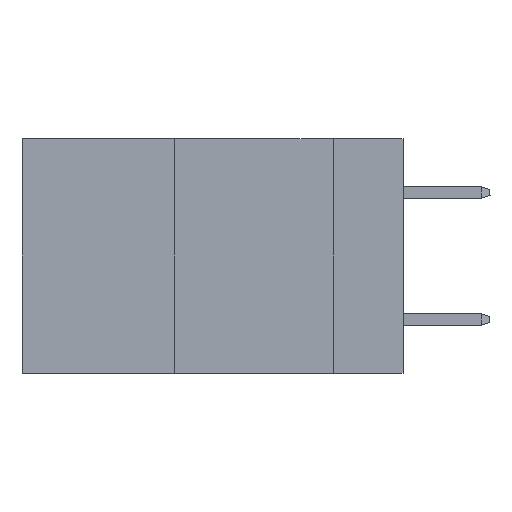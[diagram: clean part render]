
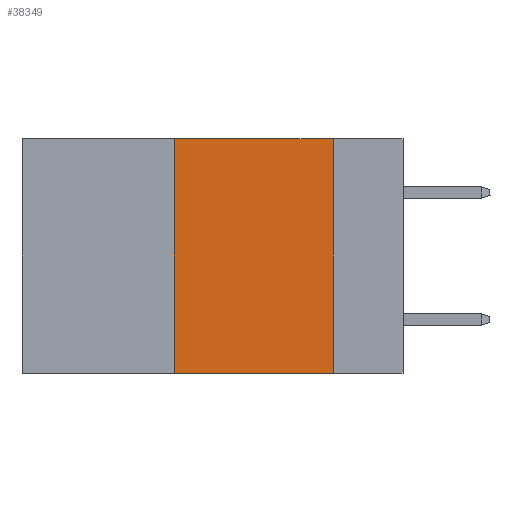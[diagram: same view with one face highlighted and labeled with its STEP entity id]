
A CAD part, left-side view. The second image highlights one B-rep face of the part: STEP entity #38349.
In plain terms, the highlighted planar face has unit normal (-1, 0, 0).
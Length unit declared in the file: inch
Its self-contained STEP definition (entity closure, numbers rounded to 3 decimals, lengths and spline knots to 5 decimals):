
#285 = ORIENTED_EDGE ( 'NONE', *, *, #9328, .T. ) ;
#897 = CARTESIAN_POINT ( 'NONE',  ( 0., 0.11, 0. ) ) ;
#1718 = VECTOR ( 'NONE', #2829, 39.37008 ) ;
#2829 = DIRECTION ( 'NONE',  ( 0., -1., 0. ) ) ;
#4061 = DIRECTION ( 'NONE',  ( 1., 0., 0. ) ) ;
#5823 = DIRECTION ( 'NONE',  ( 0., 0., 1. ) ) ;
#6064 = CARTESIAN_POINT ( 'NONE',  ( 0., 0.36, 0. ) ) ;
#6321 = VERTEX_POINT ( 'NONE', #897 ) ;
#6685 = CARTESIAN_POINT ( 'NONE',  ( 0., 0.36, 0. ) ) ;
#8329 = CARTESIAN_POINT ( 'NONE',  ( 0., 0.6, 0. ) ) ;
#8340 = CARTESIAN_POINT ( 'NONE',  ( 0., 0.11, -0.37 ) ) ;
#8440 = VERTEX_POINT ( 'NONE', #26743 ) ;
#9328 = EDGE_CURVE ( 'NONE', #8440, #16911, #39253, .T. ) ;
#11357 = DIRECTION ( 'NONE',  ( 0., 0., -1. ) ) ;
#14719 = FACE_OUTER_BOUND ( 'NONE', #33033, .T. ) ;
#16499 = EDGE_CURVE ( 'NONE', #8440, #18585, #27215, .T. ) ;
#16911 = VERTEX_POINT ( 'NONE', #8340 ) ;
#18585 = VERTEX_POINT ( 'NONE', #6685 ) ;
#19195 = VECTOR ( 'NONE', #5823, 39.37008 ) ;
#21562 = PLANE ( 'NONE',  #39995 ) ;
#21683 = ORIENTED_EDGE ( 'NONE', *, *, #16499, .F. ) ;
#25101 = ORIENTED_EDGE ( 'NONE', *, *, #29028, .F. ) ;
#26743 = CARTESIAN_POINT ( 'NONE',  ( 0., 0.36, -0.37 ) ) ;
#27215 = LINE ( 'NONE', #6064, #19195 ) ;
#27811 = LINE ( 'NONE', #37374, #1718 ) ;
#29028 = EDGE_CURVE ( 'NONE', #6321, #16911, #39542, .T. ) ;
#29329 = CARTESIAN_POINT ( 'NONE',  ( 0., 0.11, 0. ) ) ;
#31475 = EDGE_CURVE ( 'NONE', #18585, #6321, #27811, .T. ) ;
#32652 = CARTESIAN_POINT ( 'NONE',  ( 0., 0.6, -0.37 ) ) ;
#33033 = EDGE_LOOP ( 'NONE', ( #25101, #34110, #21683, #285 ) ) ;
#34110 = ORIENTED_EDGE ( 'NONE', *, *, #31475, .F. ) ;
#35880 = DIRECTION ( 'NONE',  ( 0., 0., -1. ) ) ;
#36535 = VECTOR ( 'NONE', #39033, 39.37008 ) ;
#37374 = CARTESIAN_POINT ( 'NONE',  ( 0., 0.6, 0. ) ) ;
#38349 = ADVANCED_FACE ( 'NONE', ( #14719 ), #21562, .F. ) ;
#39033 = DIRECTION ( 'NONE',  ( 0., -1., 0. ) ) ;
#39253 = LINE ( 'NONE', #32652, #36535 ) ;
#39542 = LINE ( 'NONE', #29329, #40769 ) ;
#39995 = AXIS2_PLACEMENT_3D ( 'NONE', #8329, #4061, #35880 ) ;
#40769 = VECTOR ( 'NONE', #11357, 39.37008 ) ;
